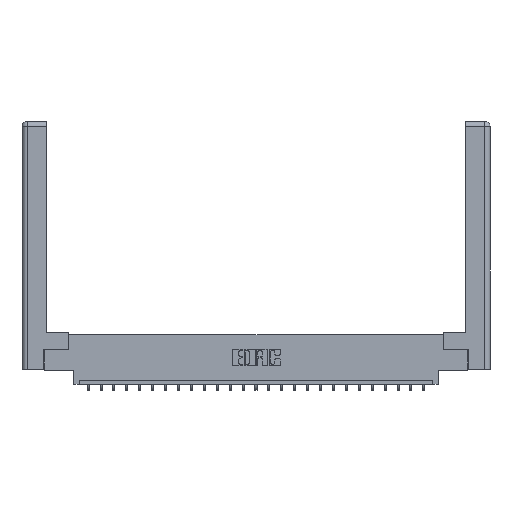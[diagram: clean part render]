
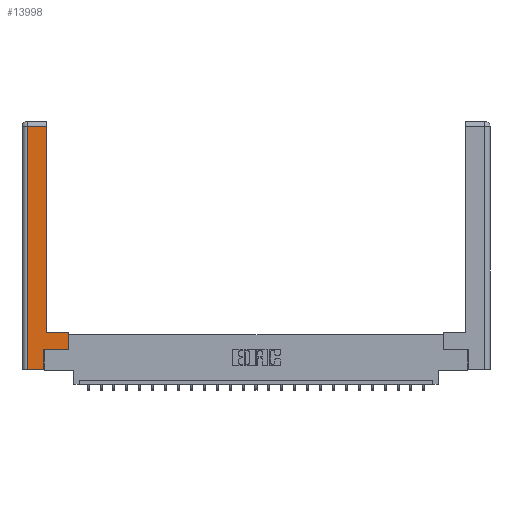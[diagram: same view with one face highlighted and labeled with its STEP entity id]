
A CAD part, top view. The second image highlights one B-rep face of the part: STEP entity #13998.
In plain terms, the highlighted planar face has unit normal (0, 0, 1).
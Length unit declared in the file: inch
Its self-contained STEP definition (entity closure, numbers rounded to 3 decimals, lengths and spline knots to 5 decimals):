
#7 = LINE ( 'NONE', #19964, #5986 ) ;
#574 = DIRECTION ( 'NONE',  ( -1., 0., 0. ) ) ;
#1111 = LINE ( 'NONE', #3385, #6530 ) ;
#1524 = CARTESIAN_POINT ( 'NONE',  ( 0.0615, 0., 0. ) ) ;
#1640 = VERTEX_POINT ( 'NONE', #2335 ) ;
#2335 = CARTESIAN_POINT ( 'NONE',  ( 0.295, 2.94, 0. ) ) ;
#2521 = ORIENTED_EDGE ( 'NONE', *, *, #14205, .T. ) ;
#3036 = EDGE_CURVE ( 'NONE', #1640, #3356, #20931, .T. ) ;
#3243 = ORIENTED_EDGE ( 'NONE', *, *, #7253, .T. ) ;
#3356 = VERTEX_POINT ( 'NONE', #5090 ) ;
#3378 = ORIENTED_EDGE ( 'NONE', *, *, #3036, .T. ) ;
#3385 = CARTESIAN_POINT ( 'NONE',  ( 0.565, 0.245, 0. ) ) ;
#4176 = VECTOR ( 'NONE', #22982, 39.37008 ) ;
#4564 = EDGE_CURVE ( 'NONE', #6313, #9187, #21427, .T. ) ;
#4607 = EDGE_LOOP ( 'NONE', ( #23814, #3378, #17476, #2521, #7741, #9821, #10019, #3243 ) ) ;
#4910 = VECTOR ( 'NONE', #15803, 39.37008 ) ;
#5090 = CARTESIAN_POINT ( 'NONE',  ( 0.0615, 2.94, 0. ) ) ;
#5741 = VERTEX_POINT ( 'NONE', #14845 ) ;
#5986 = VECTOR ( 'NONE', #6459, 39.37008 ) ;
#6313 = VERTEX_POINT ( 'NONE', #14515 ) ;
#6459 = DIRECTION ( 'NONE',  ( 0., 1., 0. ) ) ;
#6530 = VECTOR ( 'NONE', #11040, 39.37008 ) ;
#7253 = EDGE_CURVE ( 'NONE', #8574, #22929, #10924, .T. ) ;
#7655 = AXIS2_PLACEMENT_3D ( 'NONE', #12066, #23542, #574 ) ;
#7741 = ORIENTED_EDGE ( 'NONE', *, *, #4564, .T. ) ;
#7809 = CARTESIAN_POINT ( 'NONE',  ( 0.0615, 0., 0. ) ) ;
#7963 = DIRECTION ( 'NONE',  ( 0., 1., 0. ) ) ;
#8105 = CARTESIAN_POINT ( 'NONE',  ( 0.265, 0., 0. ) ) ;
#8574 = VERTEX_POINT ( 'NONE', #13895 ) ;
#9187 = VERTEX_POINT ( 'NONE', #23977 ) ;
#9257 = EDGE_CURVE ( 'NONE', #3356, #23527, #12622, .T. ) ;
#9821 = ORIENTED_EDGE ( 'NONE', *, *, #10661, .T. ) ;
#10019 = ORIENTED_EDGE ( 'NONE', *, *, #12904, .T. ) ;
#10612 = CARTESIAN_POINT ( 'NONE',  ( 0.295, 3., 0. ) ) ;
#10661 = EDGE_CURVE ( 'NONE', #9187, #5741, #1111, .T. ) ;
#10734 = VECTOR ( 'NONE', #12706, 39.37008 ) ;
#10924 = LINE ( 'NONE', #13600, #4910 ) ;
#11040 = DIRECTION ( 'NONE',  ( 1., 0., 0. ) ) ;
#12066 = CARTESIAN_POINT ( 'NONE',  ( 0., 0., 0. ) ) ;
#12622 = LINE ( 'NONE', #7809, #4176 ) ;
#12706 = DIRECTION ( 'NONE',  ( -1., 0., 0. ) ) ;
#12847 = FACE_OUTER_BOUND ( 'NONE', #4607, .T. ) ;
#12904 = EDGE_CURVE ( 'NONE', #5741, #8574, #7, .T. ) ;
#13600 = CARTESIAN_POINT ( 'NONE',  ( 0.295, 0.45, 0. ) ) ;
#13675 = CARTESIAN_POINT ( 'NONE',  ( 0.265, 0.245, 0. ) ) ;
#13895 = CARTESIAN_POINT ( 'NONE',  ( 0.565, 0.45, 0. ) ) ;
#13919 = PLANE ( 'NONE',  #7655 ) ;
#13970 = DIRECTION ( 'NONE',  ( 1., 0., 0. ) ) ;
#13998 = ADVANCED_FACE ( 'NONE', ( #12847 ), #13919, .F. ) ;
#14205 = EDGE_CURVE ( 'NONE', #23527, #6313, #24547, .T. ) ;
#14515 = CARTESIAN_POINT ( 'NONE',  ( 0.265, 0., 0. ) ) ;
#14845 = CARTESIAN_POINT ( 'NONE',  ( 0.565, 0.245, 0. ) ) ;
#15803 = DIRECTION ( 'NONE',  ( -1., 0., 0. ) ) ;
#16085 = VECTOR ( 'NONE', #7963, 39.37008 ) ;
#17472 = CARTESIAN_POINT ( 'NONE',  ( 0.295, 0.45, 0. ) ) ;
#17476 = ORIENTED_EDGE ( 'NONE', *, *, #9257, .T. ) ;
#17509 = VECTOR ( 'NONE', #24026, 39.37008 ) ;
#19436 = VECTOR ( 'NONE', #13970, 39.37008 ) ;
#19964 = CARTESIAN_POINT ( 'NONE',  ( 0.565, 0.45, 0. ) ) ;
#20181 = LINE ( 'NONE', #10612, #17509 ) ;
#20931 = LINE ( 'NONE', #23856, #10734 ) ;
#21427 = LINE ( 'NONE', #13675, #16085 ) ;
#22929 = VERTEX_POINT ( 'NONE', #17472 ) ;
#22982 = DIRECTION ( 'NONE',  ( 0., -1., 0. ) ) ;
#23527 = VERTEX_POINT ( 'NONE', #1524 ) ;
#23542 = DIRECTION ( 'NONE',  ( 0., 0., -1. ) ) ;
#23814 = ORIENTED_EDGE ( 'NONE', *, *, #23889, .T. ) ;
#23856 = CARTESIAN_POINT ( 'NONE',  ( 0.0615, 2.94, 0. ) ) ;
#23889 = EDGE_CURVE ( 'NONE', #22929, #1640, #20181, .T. ) ;
#23977 = CARTESIAN_POINT ( 'NONE',  ( 0.265, 0.245, 0. ) ) ;
#24026 = DIRECTION ( 'NONE',  ( 0., 1., 0. ) ) ;
#24547 = LINE ( 'NONE', #8105, #19436 ) ;
